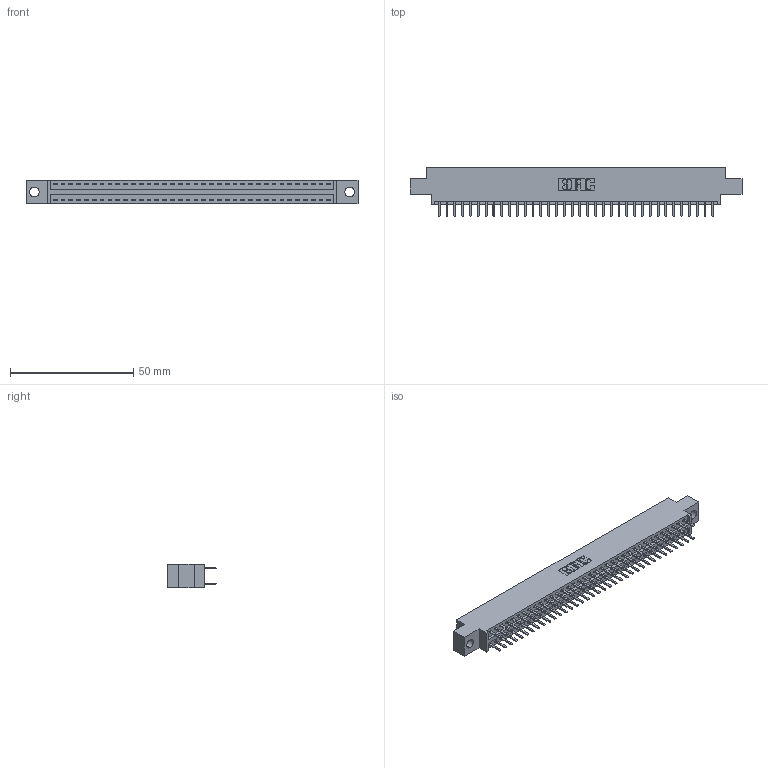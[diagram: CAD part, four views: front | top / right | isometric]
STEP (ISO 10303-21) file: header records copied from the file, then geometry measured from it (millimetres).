
FILE_DESCRIPTION (( 'STEP AP203' ), '1' );
FILE_NAME ('396-072-520-804.STEP', '2019-11-02T11:03:08', ( '' ), ( '' ), 'SwSTEP 2.0', 'SolidWorks 2016', '' );
FILE_SCHEMA (( 'CONFIG_CONTROL_DESIGN' ));
Length unit declared in the file: inch
Products named in the file (3): 346 Part_0.170 Offset - 0.156 Dia-TH; 345-292-001_345-293-120; 396-072-520-804
Assembly tree (73 placements, depth 2):
  396-072-520-804
    346 Part_0.170 Offset - 0.156 Dia-TH
    345-292-001_345-293-120  x72
Bounding box: 134.87 x 20.02 x 9.4 mm (x, y, z)
Volume: 12831.2 mm3; surface area: 17461.8 mm2
Topology: 73 solids, 73 shells, 4158 faces, 12077 edges, 7858 vertices
Faces by surface type: plane 2744, cylinder 1414
Entity records: 24551 total; most frequent: CARTESIAN_POINT 4068, ORIENTED_EDGE 3990, DIRECTION 3623, EDGE_CURVE 1995, LINE 1715, VECTOR 1715, VERTEX_POINT 1326, AXIS2_PLACEMENT_3D 954
